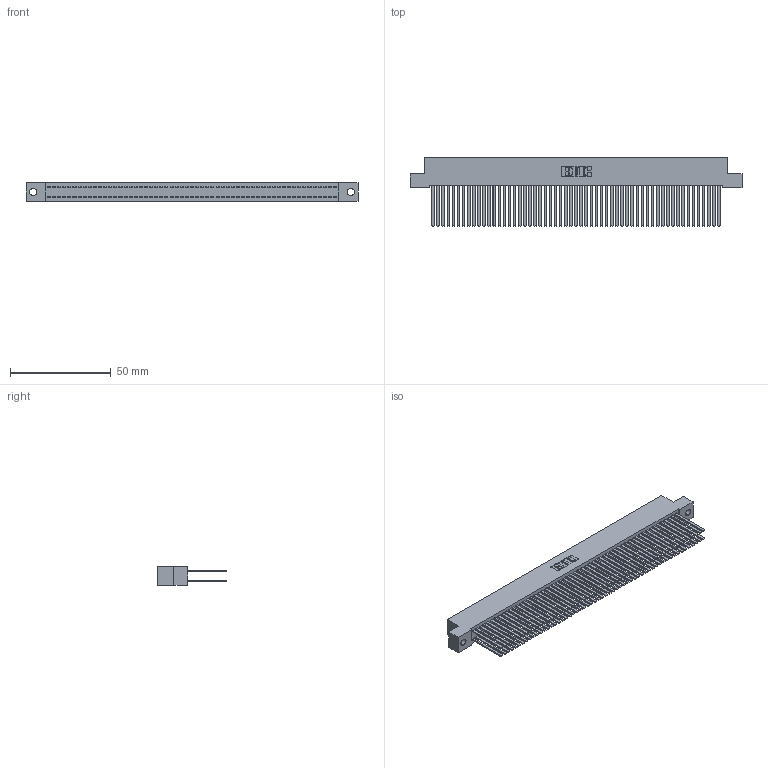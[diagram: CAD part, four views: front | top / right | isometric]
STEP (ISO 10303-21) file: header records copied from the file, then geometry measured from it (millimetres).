
FILE_DESCRIPTION (( 'STEP AP203' ), '1' );
FILE_NAME ('392-114-544-202.STEP', '2019-10-10T01:10:04', ( '' ), ( '' ), 'SwSTEP 2.0', 'SolidWorks 2016', '' );
FILE_SCHEMA (( 'CONFIG_CONTROL_DESIGN' ));
Length unit declared in the file: inch
Products named in the file (3): 392-114-544-202; 342 Part_.128 Slot; 345-292-001_345-293-144
Assembly tree (115 placements, depth 2):
  392-114-544-202
    342 Part_.128 Slot
    345-292-001_345-293-144  x114
Bounding box: 165.1 x 34.3 x 9.4 mm (x, y, z)
Volume: 16451.1 mm3; surface area: 31333 mm2
Topology: 115 solids, 115 shells, 5358 faces, 15929 edges, 10466 vertices
Faces by surface type: plane 3718, cylinder 1640
Entity records: 34549 total; most frequent: CARTESIAN_POINT 5706, ORIENTED_EDGE 5642, DIRECTION 4845, EDGE_CURVE 2821, LINE 2697, VECTOR 2697, VERTEX_POINT 1878, AXIS2_PLACEMENT_3D 1074
